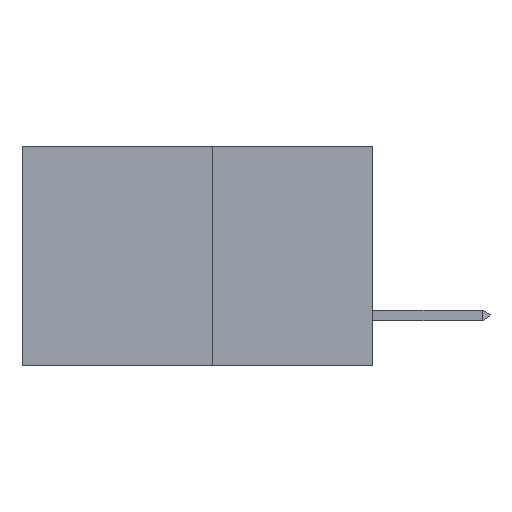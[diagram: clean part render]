
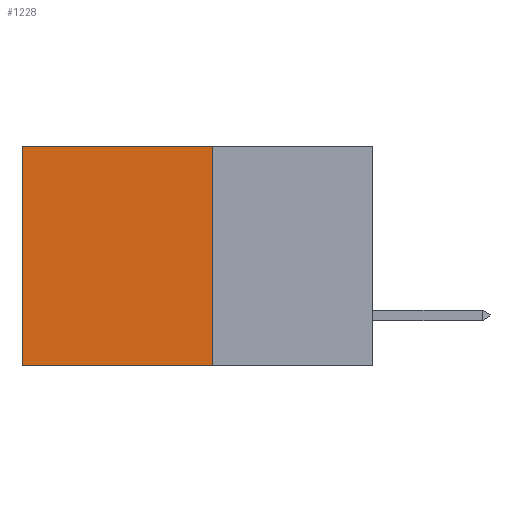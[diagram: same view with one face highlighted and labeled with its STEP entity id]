
A CAD part, left-side view. The second image highlights one B-rep face of the part: STEP entity #1228.
In plain terms, the highlighted planar face has unit normal (-1, 0, 0).
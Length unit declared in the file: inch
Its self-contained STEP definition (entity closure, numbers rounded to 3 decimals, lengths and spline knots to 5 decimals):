
#221 = DIRECTION ( 'NONE',  ( 0., 0., -1. ) ) ;
#1143 = VECTOR ( 'NONE', #4845, 39.37008 ) ;
#1228 = ADVANCED_FACE ( 'NONE', ( #17869 ), #12342, .F. ) ;
#1967 = DIRECTION ( 'NONE',  ( 0., 0., -1. ) ) ;
#2008 = DIRECTION ( 'NONE',  ( 1., 0., 0. ) ) ;
#2167 = VERTEX_POINT ( 'NONE', #10005 ) ;
#2922 = DIRECTION ( 'NONE',  ( 0., 0., -1. ) ) ;
#3127 = CARTESIAN_POINT ( 'NONE',  ( 0.277, 0.27, -0.37 ) ) ;
#3170 = ORIENTED_EDGE ( 'NONE', *, *, #12612, .T. ) ;
#3191 = EDGE_LOOP ( 'NONE', ( #14119, #5371, #9819, #3170 ) ) ;
#3260 = EDGE_CURVE ( 'NONE', #7596, #7354, #16138, .T. ) ;
#3399 = LINE ( 'NONE', #3127, #18277 ) ;
#4845 = DIRECTION ( 'NONE',  ( 0., 1., 0. ) ) ;
#4919 = VECTOR ( 'NONE', #2922, 39.37008 ) ;
#5365 = LINE ( 'NONE', #17287, #4919 ) ;
#5371 = ORIENTED_EDGE ( 'NONE', *, *, #3260, .F. ) ;
#6346 = CARTESIAN_POINT ( 'NONE',  ( 0.277, 0.59, 0. ) ) ;
#6868 = DIRECTION ( 'NONE',  ( 0., 1., 0. ) ) ;
#7354 = VERTEX_POINT ( 'NONE', #13716 ) ;
#7596 = VERTEX_POINT ( 'NONE', #12845 ) ;
#9756 = CARTESIAN_POINT ( 'NONE',  ( 0.277, 0.27, -0.37 ) ) ;
#9819 = ORIENTED_EDGE ( 'NONE', *, *, #12478, .F. ) ;
#10005 = CARTESIAN_POINT ( 'NONE',  ( 0.277, 0.27, 0. ) ) ;
#10631 = CARTESIAN_POINT ( 'NONE',  ( 0.277, 0.27, 0. ) ) ;
#11841 = VECTOR ( 'NONE', #6868, 39.37008 ) ;
#12342 = PLANE ( 'NONE',  #15780 ) ;
#12478 = EDGE_CURVE ( 'NONE', #2167, #7596, #3399, .T. ) ;
#12612 = EDGE_CURVE ( 'NONE', #2167, #17277, #12652, .T. ) ;
#12652 = LINE ( 'NONE', #10631, #1143 ) ;
#12845 = CARTESIAN_POINT ( 'NONE',  ( 0.277, 0.27, -0.37 ) ) ;
#13716 = CARTESIAN_POINT ( 'NONE',  ( 0.277, 0.59, -0.37 ) ) ;
#14119 = ORIENTED_EDGE ( 'NONE', *, *, #14859, .T. ) ;
#14859 = EDGE_CURVE ( 'NONE', #17277, #7354, #5365, .T. ) ;
#15780 = AXIS2_PLACEMENT_3D ( 'NONE', #15824, #2008, #1967 ) ;
#15824 = CARTESIAN_POINT ( 'NONE',  ( 0.277, 0.27, -0.37 ) ) ;
#16138 = LINE ( 'NONE', #9756, #11841 ) ;
#17277 = VERTEX_POINT ( 'NONE', #6346 ) ;
#17287 = CARTESIAN_POINT ( 'NONE',  ( 0.277, 0.59, -0.37 ) ) ;
#17869 = FACE_OUTER_BOUND ( 'NONE', #3191, .T. ) ;
#18277 = VECTOR ( 'NONE', #221, 39.37008 ) ;
